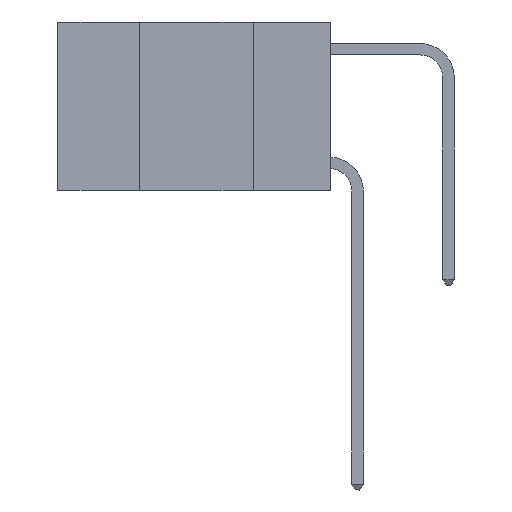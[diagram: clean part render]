
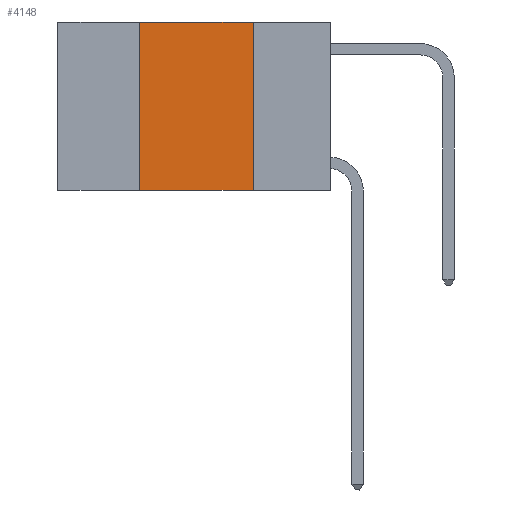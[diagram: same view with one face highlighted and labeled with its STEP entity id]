
A CAD part, left-side view. The second image highlights one B-rep face of the part: STEP entity #4148.
In plain terms, the highlighted planar face has unit normal (-1, 0, 0).
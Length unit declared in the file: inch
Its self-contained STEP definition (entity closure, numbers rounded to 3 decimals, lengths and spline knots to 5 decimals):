
#551 = LINE ( 'NONE', #8556, #1659 ) ;
#1659 = VECTOR ( 'NONE', #15721, 39.37008 ) ;
#1802 = VERTEX_POINT ( 'NONE', #3654 ) ;
#2704 = VECTOR ( 'NONE', #9863, 39.37008 ) ;
#3265 = VERTEX_POINT ( 'NONE', #26641 ) ;
#3559 = LINE ( 'NONE', #8039, #12849 ) ;
#3654 = CARTESIAN_POINT ( 'NONE',  ( 0., 0.42, -0.37 ) ) ;
#4148 = ADVANCED_FACE ( 'NONE', ( #8647 ), #10177, .F. ) ;
#5829 = AXIS2_PLACEMENT_3D ( 'NONE', #17481, #17274, #22189 ) ;
#5890 = DIRECTION ( 'NONE',  ( 0., 0., 1. ) ) ;
#7271 = CARTESIAN_POINT ( 'NONE',  ( 0., 0.17, 0. ) ) ;
#8039 = CARTESIAN_POINT ( 'NONE',  ( 0., 0.42, 0. ) ) ;
#8556 = CARTESIAN_POINT ( 'NONE',  ( 0., 0.6, -0.37 ) ) ;
#8647 = FACE_OUTER_BOUND ( 'NONE', #12389, .T. ) ;
#9863 = DIRECTION ( 'NONE',  ( 0., 0., -1. ) ) ;
#10177 = PLANE ( 'NONE',  #5829 ) ;
#10982 = ORIENTED_EDGE ( 'NONE', *, *, #11702, .F. ) ;
#11227 = CARTESIAN_POINT ( 'NONE',  ( 0., 0.42, 0. ) ) ;
#11702 = EDGE_CURVE ( 'NONE', #23079, #3265, #12191, .T. ) ;
#12191 = LINE ( 'NONE', #14079, #28312 ) ;
#12323 = VERTEX_POINT ( 'NONE', #25812 ) ;
#12389 = EDGE_LOOP ( 'NONE', ( #19319, #10982, #19836, #15241 ) ) ;
#12849 = VECTOR ( 'NONE', #5890, 39.37008 ) ;
#14079 = CARTESIAN_POINT ( 'NONE',  ( 0., 0.6, 0. ) ) ;
#14089 = EDGE_CURVE ( 'NONE', #3265, #12323, #15405, .T. ) ;
#15241 = ORIENTED_EDGE ( 'NONE', *, *, #28579, .T. ) ;
#15405 = LINE ( 'NONE', #7271, #2704 ) ;
#15721 = DIRECTION ( 'NONE',  ( 0., -1., 0. ) ) ;
#17274 = DIRECTION ( 'NONE',  ( 1., 0., 0. ) ) ;
#17481 = CARTESIAN_POINT ( 'NONE',  ( 0., 0.6, 0. ) ) ;
#19319 = ORIENTED_EDGE ( 'NONE', *, *, #14089, .F. ) ;
#19836 = ORIENTED_EDGE ( 'NONE', *, *, #30706, .F. ) ;
#22189 = DIRECTION ( 'NONE',  ( 0., 0., -1. ) ) ;
#23079 = VERTEX_POINT ( 'NONE', #11227 ) ;
#23675 = DIRECTION ( 'NONE',  ( 0., -1., 0. ) ) ;
#25812 = CARTESIAN_POINT ( 'NONE',  ( 0., 0.17, -0.37 ) ) ;
#26641 = CARTESIAN_POINT ( 'NONE',  ( 0., 0.17, 0. ) ) ;
#28312 = VECTOR ( 'NONE', #23675, 39.37008 ) ;
#28579 = EDGE_CURVE ( 'NONE', #1802, #12323, #551, .T. ) ;
#30706 = EDGE_CURVE ( 'NONE', #1802, #23079, #3559, .T. ) ;
